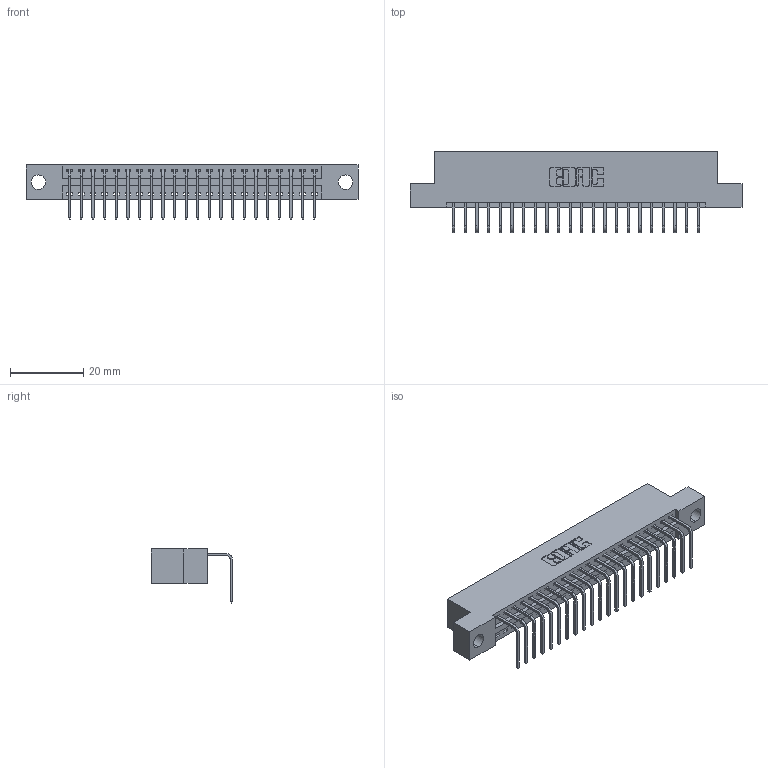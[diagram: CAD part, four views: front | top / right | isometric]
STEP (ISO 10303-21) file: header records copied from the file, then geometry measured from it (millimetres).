
FILE_DESCRIPTION (( 'STEP AP203' ), '1' );
FILE_NAME ('346-022-558-104.STEP', '2022-05-05T20:04:59', ( '' ), ( '' ), 'SwSTEP 2.0', 'SolidWorks 2020', '' );
FILE_SCHEMA (( 'CONFIG_CONTROL_DESIGN' ));
Length unit declared in the file: inch
Products named in the file (3): 345-292-001_558 Tail - 2; 346 Part_Flush Mounting Lugs - 0.156 Dia-TH; 346-022-558-104
Assembly tree (23 placements, depth 2):
  346-022-558-104
    346 Part_Flush Mounting Lugs - 0.156 Dia-TH
    345-292-001_558 Tail - 2  x22
Bounding box: 90.42 x 22.16 x 14.73 mm (x, y, z)
Volume: 8485.1 mm3; surface area: 10664 mm2
Topology: 23 solids, 23 shells, 1456 faces, 4369 edges, 2882 vertices
Faces by surface type: plane 1014, cylinder 442
Entity records: 16849 total; most frequent: CARTESIAN_POINT 2904, ORIENTED_EDGE 2858, DIRECTION 2585, EDGE_CURVE 1429, LINE 1209, VECTOR 1209, VERTEX_POINT 950, AXIS2_PLACEMENT_3D 688
